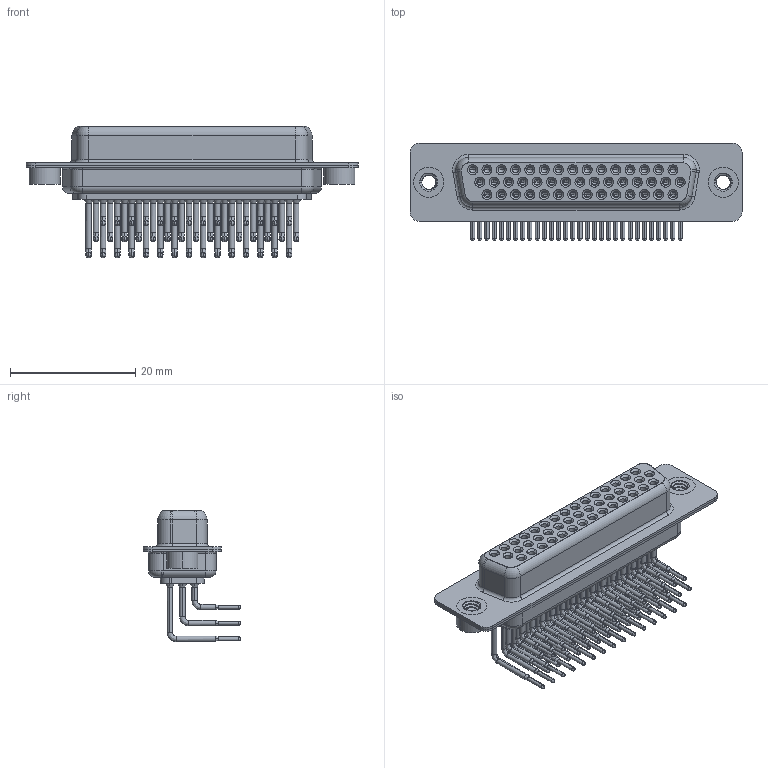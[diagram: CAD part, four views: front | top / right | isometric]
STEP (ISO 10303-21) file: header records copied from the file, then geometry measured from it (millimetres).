
FILE_DESCRIPTION (( 'STEP AP203' ), '1' );
FILE_NAME ('634-M44-363-WN2.STEP', '2018-09-28T01:15:10', ( '' ), ( '' ), 'SwSTEP 2.0', 'SolidWorks 2016', '' );
FILE_SCHEMA (( 'CONFIG_CONTROL_DESIGN' ));
Length unit declared in the file: millimetre
Products named in the file (8): 634M Contact Row 2; 634M Contact Row 3; 634M 4-40 Threaded Rivet; 634-M44-363-WN2; 634M Housing_44 Contacts; 634M Shell Front_44 Contacts; 634M Shell Rear_44 Contacts; 634M Contact Row 1
Assembly tree (49 placements, depth 2):
  634-M44-363-WN2
    634M Housing_44 Contacts
    634M Shell Front_44 Contacts
    634M Shell Rear_44 Contacts
    634M Contact Row 1  x15
    634M Contact Row 2  x15
    634M Contact Row 3  x14
    634M 4-40 Threaded Rivet  x2
Bounding box: 53.05 x 15.6 x 21.02 mm (x, y, z)
Volume: 3837.5 mm3; surface area: 13038 mm2
Topology: 49 solids, 49 shells, 2611 faces, 6627 edges, 4169 vertices
Faces by surface type: cylinder 1149, plane 727, cone 490, bspline 182, torus 63
Entity records: 30871 total; most frequent: CARTESIAN_POINT 6443, DIRECTION 5225, ORIENTED_EDGE 4292, AXIS2_PLACEMENT_3D 2207, EDGE_CURVE 2146, VERTEX_POINT 1369, CIRCLE 1232, EDGE_LOOP 1187
